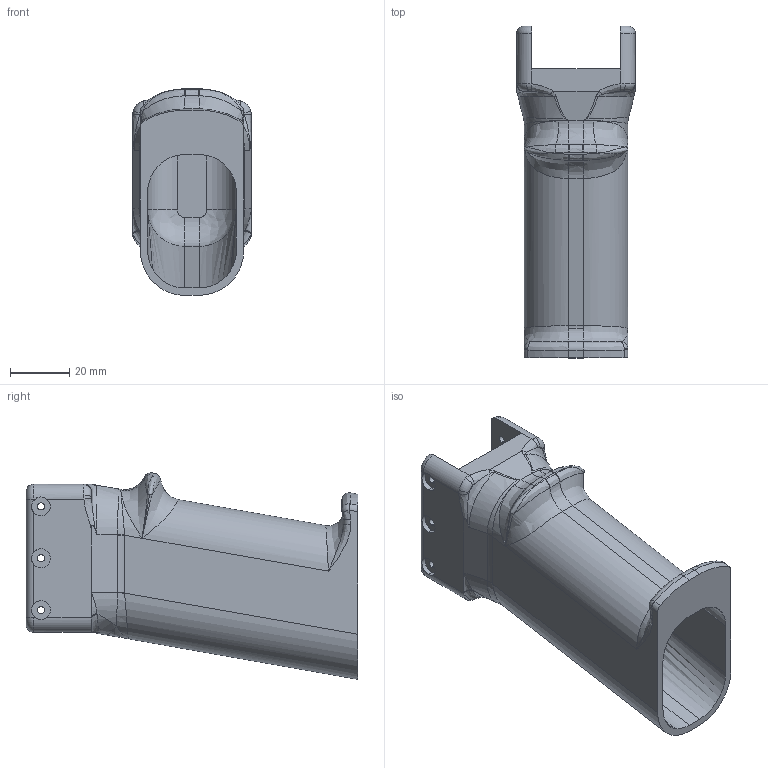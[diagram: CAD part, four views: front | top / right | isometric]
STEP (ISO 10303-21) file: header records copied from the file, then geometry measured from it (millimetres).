
FILE_DESCRIPTION (( 'STEP AP203' ), '1' );
FILE_NAME ('Handle.STEP', '2013-11-14T05:09:47', ( '' ), ( '' ), 'SwSTEP 2.0', 'SolidWorks 2013', '' );
FILE_SCHEMA (( 'CONFIG_CONTROL_DESIGN' ));
Length unit declared in the file: millimetre
Products named in the file (1): Handle
Bounding box: 40 x 112 x 69.76 mm (x, y, z)
Volume: 63406.7 mm3; surface area: 33283.7 mm2
Topology: 1 solids, 1 shells, 195 faces, 496 edges, 290 vertices
Faces by surface type: bspline 93, cylinder 51, plane 41, torus 6, sphere 4
Entity records: 14298 total; most frequent: CARTESIAN_POINT 10299, ORIENTED_EDGE 958, DIRECTION 626, EDGE_CURVE 479, VERTEX_POINT 287, AXIS2_PLACEMENT_3D 251, EDGE_LOOP 208, ADVANCED_FACE 195
